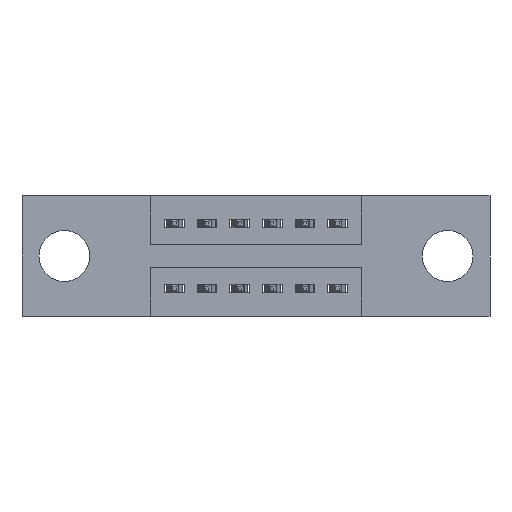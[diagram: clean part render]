
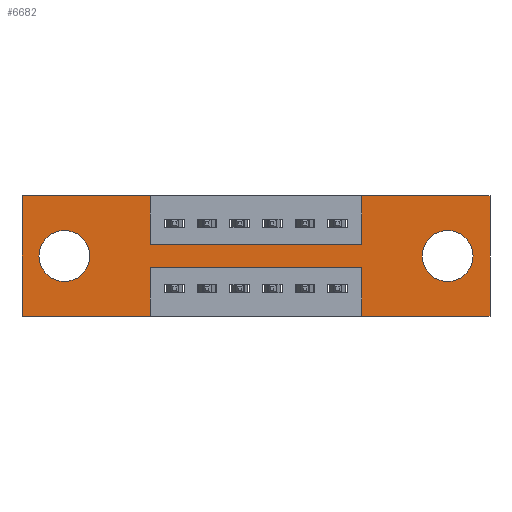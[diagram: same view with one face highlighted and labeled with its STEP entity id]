
A CAD part, front view. The second image highlights one B-rep face of the part: STEP entity #6682.
In plain terms, the highlighted planar face has unit normal (0, -1, 0).
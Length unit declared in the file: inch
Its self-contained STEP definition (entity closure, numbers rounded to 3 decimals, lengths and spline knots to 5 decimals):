
#18 = CARTESIAN_POINT ( 'NONE',  ( 1.0425, 0., -0.37 ) ) ;
#139 = DIRECTION ( 'NONE',  ( 1., 0., 0. ) ) ;
#346 = CARTESIAN_POINT ( 'NONE',  ( 0., 0., -0.37 ) ) ;
#391 = LINE ( 'NONE', #6404, #5164 ) ;
#449 = EDGE_CURVE ( 'NONE', #4921, #8897, #4023, .T. ) ;
#493 = CARTESIAN_POINT ( 'NONE',  ( 0.3925, 0., -0.15 ) ) ;
#692 = DIRECTION ( 'NONE',  ( 0., 0., -1. ) ) ;
#764 = ORIENTED_EDGE ( 'NONE', *, *, #6995, .F. ) ;
#785 = EDGE_LOOP ( 'NONE', ( #3272, #1663 ) ) ;
#797 = ORIENTED_EDGE ( 'NONE', *, *, #8191, .F. ) ;
#1018 = CARTESIAN_POINT ( 'NONE',  ( 1.0425, 0., 0. ) ) ;
#1042 = ORIENTED_EDGE ( 'NONE', *, *, #3651, .F. ) ;
#1083 = ORIENTED_EDGE ( 'NONE', *, *, #4338, .T. ) ;
#1149 = CARTESIAN_POINT ( 'NONE',  ( 1.0425, 0., 0. ) ) ;
#1211 = DIRECTION ( 'NONE',  ( 0., 1., 0. ) ) ;
#1238 = VERTEX_POINT ( 'NONE', #3657 ) ;
#1337 = ORIENTED_EDGE ( 'NONE', *, *, #6692, .F. ) ;
#1438 = EDGE_LOOP ( 'NONE', ( #4585, #6145, #1042, #3466, #5610, #7705, #7722, #764, #4779, #797, #4841, #1337 ) ) ;
#1463 = CARTESIAN_POINT ( 'NONE',  ( 1.305, 0., -0.185 ) ) ;
#1505 = CARTESIAN_POINT ( 'NONE',  ( 0., 0., 0. ) ) ;
#1522 = CIRCLE ( 'NONE', #7186, 0.078 ) ;
#1663 = ORIENTED_EDGE ( 'NONE', *, *, #4518, .T. ) ;
#1686 = EDGE_CURVE ( 'NONE', #6875, #4921, #391, .T. ) ;
#1704 = FACE_BOUND ( 'NONE', #5545, .T. ) ;
#1757 = FACE_OUTER_BOUND ( 'NONE', #1438, .T. ) ;
#1788 = VERTEX_POINT ( 'NONE', #493 ) ;
#1803 = DIRECTION ( 'NONE',  ( -1., 0., 0. ) ) ;
#1854 = CARTESIAN_POINT ( 'NONE',  ( 1.0425, 0., -0.37 ) ) ;
#1958 = CARTESIAN_POINT ( 'NONE',  ( 0.3925, 0., 0. ) ) ;
#2285 = CARTESIAN_POINT ( 'NONE',  ( 0., 0., 0. ) ) ;
#2300 = DIRECTION ( 'NONE',  ( 0., 0., 1. ) ) ;
#2324 = DIRECTION ( 'NONE',  ( 0., 0., -1. ) ) ;
#2334 = VERTEX_POINT ( 'NONE', #6904 ) ;
#2593 = VERTEX_POINT ( 'NONE', #1018 ) ;
#2623 = EDGE_CURVE ( 'NONE', #2334, #8273, #8165, .T. ) ;
#2635 = CIRCLE ( 'NONE', #8954, 0.078 ) ;
#2678 = DIRECTION ( 'NONE',  ( -1., 0., 0. ) ) ;
#2731 = DIRECTION ( 'NONE',  ( 0., 0., 1. ) ) ;
#2926 = CARTESIAN_POINT ( 'NONE',  ( 1.435, 0., 0. ) ) ;
#2982 = CARTESIAN_POINT ( 'NONE',  ( 1.305, 0., -0.185 ) ) ;
#3166 = EDGE_CURVE ( 'NONE', #9468, #5452, #2635, .T. ) ;
#3272 = ORIENTED_EDGE ( 'NONE', *, *, #9367, .T. ) ;
#3279 = DIRECTION ( 'NONE',  ( 0., -1., 0. ) ) ;
#3301 = VERTEX_POINT ( 'NONE', #7176 ) ;
#3314 = DIRECTION ( 'NONE',  ( 0., 0., -1. ) ) ;
#3433 = DIRECTION ( 'NONE',  ( 0., 0., -1. ) ) ;
#3466 = ORIENTED_EDGE ( 'NONE', *, *, #2623, .F. ) ;
#3483 = CARTESIAN_POINT ( 'NONE',  ( 0., 0., 0. ) ) ;
#3537 = EDGE_CURVE ( 'NONE', #9099, #2593, #8085, .T. ) ;
#3580 = DIRECTION ( 'NONE',  ( 0., 0., 1. ) ) ;
#3651 = EDGE_CURVE ( 'NONE', #8273, #6875, #6956, .T. ) ;
#3657 = CARTESIAN_POINT ( 'NONE',  ( 1.305, 0., -0.263 ) ) ;
#3835 = DIRECTION ( 'NONE',  ( 0., 1., 0. ) ) ;
#3884 = CARTESIAN_POINT ( 'NONE',  ( 0.13, 0., -0.263 ) ) ;
#3910 = VECTOR ( 'NONE', #2300, 39.37008 ) ;
#3933 = DIRECTION ( 'NONE',  ( 1., 0., 0. ) ) ;
#3998 = VECTOR ( 'NONE', #5648, 39.37008 ) ;
#4001 = EDGE_CURVE ( 'NONE', #5132, #7972, #6175, .T. ) ;
#4014 = AXIS2_PLACEMENT_3D ( 'NONE', #1463, #4553, #692 ) ;
#4023 = LINE ( 'NONE', #5692, #5322 ) ;
#4044 = LINE ( 'NONE', #8704, #4355 ) ;
#4180 = AXIS2_PLACEMENT_3D ( 'NONE', #346, #3279, #3433 ) ;
#4194 = FACE_BOUND ( 'NONE', #785, .T. ) ;
#4314 = DIRECTION ( 'NONE',  ( -1., 0., 0. ) ) ;
#4338 = EDGE_CURVE ( 'NONE', #5452, #9468, #1522, .T. ) ;
#4353 = VECTOR ( 'NONE', #5261, 39.37008 ) ;
#4355 = VECTOR ( 'NONE', #2678, 39.37008 ) ;
#4359 = DIRECTION ( 'NONE',  ( 0., 1., 0. ) ) ;
#4492 = CARTESIAN_POINT ( 'NONE',  ( 0.3925, 0., -0.22 ) ) ;
#4518 = EDGE_CURVE ( 'NONE', #1238, #4985, #6049, .T. ) ;
#4553 = DIRECTION ( 'NONE',  ( 0., 1., 0. ) ) ;
#4585 = ORIENTED_EDGE ( 'NONE', *, *, #449, .F. ) ;
#4665 = DIRECTION ( 'NONE',  ( 0., 0., -1. ) ) ;
#4667 = EDGE_CURVE ( 'NONE', #2593, #3301, #8758, .T. ) ;
#4779 = ORIENTED_EDGE ( 'NONE', *, *, #6001, .F. ) ;
#4800 = PLANE ( 'NONE',  #4180 ) ;
#4841 = ORIENTED_EDGE ( 'NONE', *, *, #4001, .F. ) ;
#4921 = VERTEX_POINT ( 'NONE', #4492 ) ;
#4985 = VERTEX_POINT ( 'NONE', #7167 ) ;
#5132 = VERTEX_POINT ( 'NONE', #8948 ) ;
#5164 = VECTOR ( 'NONE', #1803, 39.37008 ) ;
#5261 = DIRECTION ( 'NONE',  ( 0., 0., -1. ) ) ;
#5300 = CARTESIAN_POINT ( 'NONE',  ( 1.0425, 0., -0.22 ) ) ;
#5322 = VECTOR ( 'NONE', #3314, 39.37008 ) ;
#5452 = VERTEX_POINT ( 'NONE', #8825 ) ;
#5545 = EDGE_LOOP ( 'NONE', ( #1083, #9089 ) ) ;
#5610 = ORIENTED_EDGE ( 'NONE', *, *, #9310, .F. ) ;
#5648 = DIRECTION ( 'NONE',  ( 1., 0., 0. ) ) ;
#5692 = CARTESIAN_POINT ( 'NONE',  ( 0.3925, 0., -0.37 ) ) ;
#5713 = VECTOR ( 'NONE', #3580, 39.37008 ) ;
#6001 = EDGE_CURVE ( 'NONE', #8464, #1788, #9272, .T. ) ;
#6049 = CIRCLE ( 'NONE', #9775, 0.078 ) ;
#6145 = ORIENTED_EDGE ( 'NONE', *, *, #1686, .F. ) ;
#6175 = LINE ( 'NONE', #2285, #7636 ) ;
#6404 = CARTESIAN_POINT ( 'NONE',  ( 0.3925, 0., -0.22 ) ) ;
#6407 = CARTESIAN_POINT ( 'NONE',  ( 0., 0., 0. ) ) ;
#6505 = CARTESIAN_POINT ( 'NONE',  ( 0.3925, 0., -0.15 ) ) ;
#6682 = ADVANCED_FACE ( 'NONE', ( #4194, #1704, #1757 ), #4800, .T. ) ;
#6692 = EDGE_CURVE ( 'NONE', #8897, #5132, #4044, .T. ) ;
#6875 = VERTEX_POINT ( 'NONE', #5300 ) ;
#6904 = CARTESIAN_POINT ( 'NONE',  ( 1.435, 0., -0.37 ) ) ;
#6956 = LINE ( 'NONE', #18, #3910 ) ;
#6995 = EDGE_CURVE ( 'NONE', #1788, #9099, #8797, .T. ) ;
#7020 = VECTOR ( 'NONE', #139, 39.37008 ) ;
#7089 = CARTESIAN_POINT ( 'NONE',  ( 1.0425, 0., -0.15 ) ) ;
#7167 = CARTESIAN_POINT ( 'NONE',  ( 1.305, 0., -0.107 ) ) ;
#7176 = CARTESIAN_POINT ( 'NONE',  ( 1.435, 0., 0. ) ) ;
#7186 = AXIS2_PLACEMENT_3D ( 'NONE', #8305, #1211, #7341 ) ;
#7272 = VECTOR ( 'NONE', #3933, 39.37008 ) ;
#7341 = DIRECTION ( 'NONE',  ( 0., 0., 1. ) ) ;
#7350 = CARTESIAN_POINT ( 'NONE',  ( 0., 0., -0.37 ) ) ;
#7358 = CARTESIAN_POINT ( 'NONE',  ( 0.3925, 0., -0.37 ) ) ;
#7636 = VECTOR ( 'NONE', #8418, 39.37008 ) ;
#7705 = ORIENTED_EDGE ( 'NONE', *, *, #4667, .F. ) ;
#7722 = ORIENTED_EDGE ( 'NONE', *, *, #3537, .F. ) ;
#7894 = CARTESIAN_POINT ( 'NONE',  ( 0.3925, 0., 0. ) ) ;
#7972 = VERTEX_POINT ( 'NONE', #3483 ) ;
#8085 = LINE ( 'NONE', #1149, #5713 ) ;
#8165 = LINE ( 'NONE', #7350, #9542 ) ;
#8191 = EDGE_CURVE ( 'NONE', #7972, #8464, #8449, .T. ) ;
#8273 = VERTEX_POINT ( 'NONE', #1854 ) ;
#8305 = CARTESIAN_POINT ( 'NONE',  ( 0.13, 0., -0.185 ) ) ;
#8389 = CIRCLE ( 'NONE', #4014, 0.078 ) ;
#8418 = DIRECTION ( 'NONE',  ( 0., 0., 1. ) ) ;
#8449 = LINE ( 'NONE', #1505, #7272 ) ;
#8464 = VERTEX_POINT ( 'NONE', #1958 ) ;
#8704 = CARTESIAN_POINT ( 'NONE',  ( 0., 0., -0.37 ) ) ;
#8758 = LINE ( 'NONE', #6407, #7020 ) ;
#8797 = LINE ( 'NONE', #6505, #3998 ) ;
#8825 = CARTESIAN_POINT ( 'NONE',  ( 0.13, 0., -0.107 ) ) ;
#8867 = VECTOR ( 'NONE', #4665, 39.37008 ) ;
#8897 = VERTEX_POINT ( 'NONE', #7358 ) ;
#8948 = CARTESIAN_POINT ( 'NONE',  ( 0., 0., -0.37 ) ) ;
#8954 = AXIS2_PLACEMENT_3D ( 'NONE', #9664, #4359, #2731 ) ;
#9089 = ORIENTED_EDGE ( 'NONE', *, *, #3166, .T. ) ;
#9099 = VERTEX_POINT ( 'NONE', #7089 ) ;
#9272 = LINE ( 'NONE', #7894, #8867 ) ;
#9310 = EDGE_CURVE ( 'NONE', #3301, #2334, #9861, .T. ) ;
#9367 = EDGE_CURVE ( 'NONE', #4985, #1238, #8389, .T. ) ;
#9468 = VERTEX_POINT ( 'NONE', #3884 ) ;
#9542 = VECTOR ( 'NONE', #4314, 39.37008 ) ;
#9664 = CARTESIAN_POINT ( 'NONE',  ( 0.13, 0., -0.185 ) ) ;
#9775 = AXIS2_PLACEMENT_3D ( 'NONE', #2982, #3835, #2324 ) ;
#9861 = LINE ( 'NONE', #2926, #4353 ) ;
